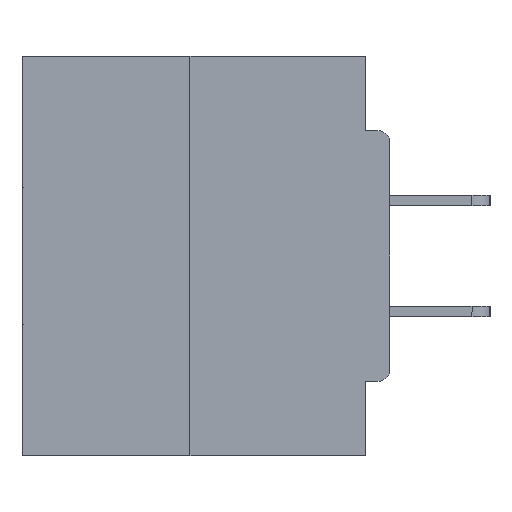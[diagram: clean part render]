
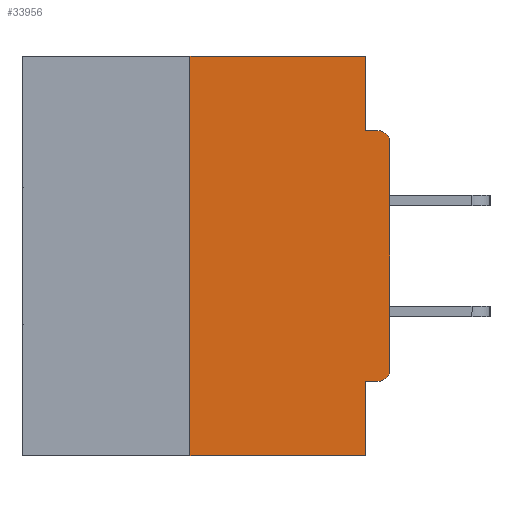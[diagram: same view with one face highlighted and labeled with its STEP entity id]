
A CAD part, left-side view. The second image highlights one B-rep face of the part: STEP entity #33956.
In plain terms, the highlighted planar face has unit normal (-1, 0, 0).
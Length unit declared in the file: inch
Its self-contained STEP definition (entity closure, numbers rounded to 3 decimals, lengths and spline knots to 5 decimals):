
#192 = CARTESIAN_POINT ( 'NONE',  ( 0., 0.46, -0.5 ) ) ;
#574 = VERTEX_POINT ( 'NONE', #31349 ) ;
#676 = ORIENTED_EDGE ( 'NONE', *, *, #24269, .T. ) ;
#1551 = LINE ( 'NONE', #31065, #4405 ) ;
#2551 = CARTESIAN_POINT ( 'NONE',  ( 0., 0.031, -0.4065 ) ) ;
#2805 = CARTESIAN_POINT ( 'NONE',  ( 0., 0., -0.1085 ) ) ;
#3021 = AXIS2_PLACEMENT_3D ( 'NONE', #22676, #10758, #4852 ) ;
#3196 = DIRECTION ( 'NONE',  ( 0., -1., 0. ) ) ;
#4004 = CARTESIAN_POINT ( 'NONE',  ( 0., 0.031, -0.5 ) ) ;
#4374 = EDGE_CURVE ( 'NONE', #25478, #15112, #6682, .T. ) ;
#4405 = VECTOR ( 'NONE', #28449, 39.37008 ) ;
#4852 = DIRECTION ( 'NONE',  ( 0., 0., -1. ) ) ;
#6682 = LINE ( 'NONE', #34255, #13748 ) ;
#7225 = ORIENTED_EDGE ( 'NONE', *, *, #21528, .F. ) ;
#7272 = ORIENTED_EDGE ( 'NONE', *, *, #20115, .T. ) ;
#7738 = CARTESIAN_POINT ( 'NONE',  ( 0., 0., -0.0935 ) ) ;
#7857 = CARTESIAN_POINT ( 'NONE',  ( 0., 0.031, 0. ) ) ;
#8072 = ORIENTED_EDGE ( 'NONE', *, *, #31426, .T. ) ;
#10677 = VECTOR ( 'NONE', #27451, 39.37008 ) ;
#10758 = DIRECTION ( 'NONE',  ( 1., 0., 0. ) ) ;
#10802 = CARTESIAN_POINT ( 'NONE',  ( 0., 0.015, -0.0935 ) ) ;
#11091 = CIRCLE ( 'NONE', #25250, 0.015 ) ;
#11179 = VERTEX_POINT ( 'NONE', #2805 ) ;
#11188 = CARTESIAN_POINT ( 'NONE',  ( 0., 0.015, -0.4065 ) ) ;
#12084 = AXIS2_PLACEMENT_3D ( 'NONE', #26550, #29554, #32564 ) ;
#13748 = VECTOR ( 'NONE', #19330, 39.37008 ) ;
#13782 = PLANE ( 'NONE',  #3021 ) ;
#14216 = CARTESIAN_POINT ( 'NONE',  ( 0., 0., -0.3915 ) ) ;
#14229 = CARTESIAN_POINT ( 'NONE',  ( 0., 0., -0.4065 ) ) ;
#14471 = VERTEX_POINT ( 'NONE', #2551 ) ;
#14575 = EDGE_CURVE ( 'NONE', #25478, #33171, #34077, .T. ) ;
#14801 = VECTOR ( 'NONE', #24971, 39.37008 ) ;
#15112 = VERTEX_POINT ( 'NONE', #17340 ) ;
#15587 = EDGE_CURVE ( 'NONE', #22332, #574, #1551, .T. ) ;
#16461 = FACE_OUTER_BOUND ( 'NONE', #34710, .T. ) ;
#16558 = VECTOR ( 'NONE', #38695, 39.37008 ) ;
#17340 = CARTESIAN_POINT ( 'NONE',  ( 0., 0.25, 0. ) ) ;
#17441 = ORIENTED_EDGE ( 'NONE', *, *, #4374, .F. ) ;
#17906 = ORIENTED_EDGE ( 'NONE', *, *, #32889, .F. ) ;
#18102 = VERTEX_POINT ( 'NONE', #11188 ) ;
#18479 = CARTESIAN_POINT ( 'NONE',  ( 0., 0.25, -0.5 ) ) ;
#19330 = DIRECTION ( 'NONE',  ( 0., 0., 1. ) ) ;
#20080 = ORIENTED_EDGE ( 'NONE', *, *, #22172, .F. ) ;
#20115 = EDGE_CURVE ( 'NONE', #11179, #31708, #11091, .T. ) ;
#20755 = CARTESIAN_POINT ( 'NONE',  ( 0., 0., 0. ) ) ;
#20771 = CARTESIAN_POINT ( 'NONE',  ( 0., 0.015, -0.1085 ) ) ;
#21148 = DIRECTION ( 'NONE',  ( -1., 0., 0. ) ) ;
#21215 = VECTOR ( 'NONE', #34204, 39.37008 ) ;
#21528 = EDGE_CURVE ( 'NONE', #15112, #22332, #38769, .T. ) ;
#21870 = VECTOR ( 'NONE', #3196, 39.37008 ) ;
#22172 = EDGE_CURVE ( 'NONE', #14471, #33171, #22740, .T. ) ;
#22332 = VERTEX_POINT ( 'NONE', #7857 ) ;
#22676 = CARTESIAN_POINT ( 'NONE',  ( 0., 0.46, 0. ) ) ;
#22740 = LINE ( 'NONE', #4004, #14801 ) ;
#22816 = ORIENTED_EDGE ( 'NONE', *, *, #32514, .F. ) ;
#23694 = ORIENTED_EDGE ( 'NONE', *, *, #15587, .F. ) ;
#24269 = EDGE_CURVE ( 'NONE', #18102, #28435, #38051, .T. ) ;
#24971 = DIRECTION ( 'NONE',  ( 0., 0., -1. ) ) ;
#25250 = AXIS2_PLACEMENT_3D ( 'NONE', #20771, #21148, #32932 ) ;
#25478 = VERTEX_POINT ( 'NONE', #18479 ) ;
#26460 = CARTESIAN_POINT ( 'NONE',  ( 0., 0.031, -0.5 ) ) ;
#26517 = VECTOR ( 'NONE', #26645, 39.37008 ) ;
#26550 = CARTESIAN_POINT ( 'NONE',  ( 0., 0.015, -0.3915 ) ) ;
#26645 = DIRECTION ( 'NONE',  ( 0., 0., 1. ) ) ;
#26845 = LINE ( 'NONE', #7738, #21215 ) ;
#27423 = CARTESIAN_POINT ( 'NONE',  ( 0., 0.46, 0. ) ) ;
#27451 = DIRECTION ( 'NONE',  ( 0., -1., 0. ) ) ;
#28435 = VERTEX_POINT ( 'NONE', #14216 ) ;
#28449 = DIRECTION ( 'NONE',  ( 0., 0., -1. ) ) ;
#29554 = DIRECTION ( 'NONE',  ( -1., 0., 0. ) ) ;
#30150 = LINE ( 'NONE', #14229, #16558 ) ;
#31065 = CARTESIAN_POINT ( 'NONE',  ( 0., 0.031, 0. ) ) ;
#31349 = CARTESIAN_POINT ( 'NONE',  ( 0., 0.031, -0.0935 ) ) ;
#31426 = EDGE_CURVE ( 'NONE', #28435, #11179, #34465, .T. ) ;
#31708 = VERTEX_POINT ( 'NONE', #10802 ) ;
#32514 = EDGE_CURVE ( 'NONE', #18102, #14471, #30150, .T. ) ;
#32564 = DIRECTION ( 'NONE',  ( 0., 0., -1. ) ) ;
#32889 = EDGE_CURVE ( 'NONE', #574, #31708, #26845, .T. ) ;
#32932 = DIRECTION ( 'NONE',  ( 0., 0., -1. ) ) ;
#33053 = ORIENTED_EDGE ( 'NONE', *, *, #14575, .T. ) ;
#33171 = VERTEX_POINT ( 'NONE', #26460 ) ;
#33956 = ADVANCED_FACE ( 'NONE', ( #16461 ), #13782, .F. ) ;
#34077 = LINE ( 'NONE', #192, #10677 ) ;
#34204 = DIRECTION ( 'NONE',  ( 0., -1., 0. ) ) ;
#34255 = CARTESIAN_POINT ( 'NONE',  ( 0., 0.25, 0. ) ) ;
#34465 = LINE ( 'NONE', #20755, #26517 ) ;
#34710 = EDGE_LOOP ( 'NONE', ( #7225, #17441, #33053, #20080, #22816, #676, #8072, #7272, #17906, #23694 ) ) ;
#38051 = CIRCLE ( 'NONE', #12084, 0.015 ) ;
#38695 = DIRECTION ( 'NONE',  ( 0., 1., 0. ) ) ;
#38769 = LINE ( 'NONE', #27423, #21870 ) ;
